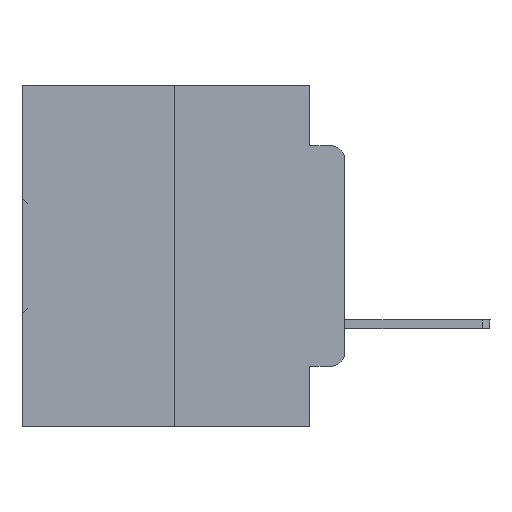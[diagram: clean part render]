
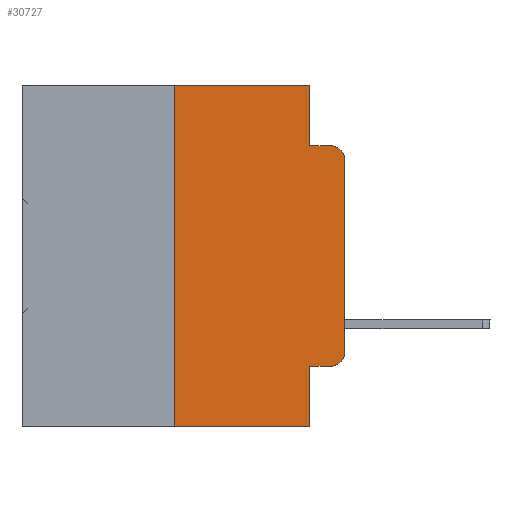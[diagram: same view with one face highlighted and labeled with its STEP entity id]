
A CAD part, left-side view. The second image highlights one B-rep face of the part: STEP entity #30727.
In plain terms, the highlighted planar face has unit normal (-1, 0, 0).
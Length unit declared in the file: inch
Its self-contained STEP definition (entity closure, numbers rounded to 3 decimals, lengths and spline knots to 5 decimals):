
#281 = LINE ( 'NONE', #11398, #8085 ) ;
#467 = ORIENTED_EDGE ( 'NONE', *, *, #11546, .F. ) ;
#2263 = VERTEX_POINT ( 'NONE', #15503 ) ;
#2699 = DIRECTION ( 'NONE',  ( 1., 0., 0. ) ) ;
#2722 = ORIENTED_EDGE ( 'NONE', *, *, #23367, .F. ) ;
#3305 = VECTOR ( 'NONE', #19633, 39.37008 ) ;
#3472 = DIRECTION ( 'NONE',  ( 0., -1., 0. ) ) ;
#3783 = CARTESIAN_POINT ( 'NONE',  ( 0., 0.25, 0. ) ) ;
#4512 = LINE ( 'NONE', #17762, #34932 ) ;
#5040 = ORIENTED_EDGE ( 'NONE', *, *, #28165, .T. ) ;
#6168 = CARTESIAN_POINT ( 'NONE',  ( 0., 0.25, 0. ) ) ;
#6306 = VERTEX_POINT ( 'NONE', #16588 ) ;
#7298 = EDGE_CURVE ( 'NONE', #8779, #32624, #9564, .T. ) ;
#7706 = AXIS2_PLACEMENT_3D ( 'NONE', #16877, #27318, #10704 ) ;
#7778 = DIRECTION ( 'NONE',  ( -1., 0., 0. ) ) ;
#7963 = EDGE_CURVE ( 'NONE', #8872, #6306, #30005, .T. ) ;
#8085 = VECTOR ( 'NONE', #22349, 39.37008 ) ;
#8494 = CARTESIAN_POINT ( 'NONE',  ( 0., 0.051, -0.4115 ) ) ;
#8779 = VERTEX_POINT ( 'NONE', #6168 ) ;
#8872 = VERTEX_POINT ( 'NONE', #8494 ) ;
#9047 = VECTOR ( 'NONE', #26353, 39.37008 ) ;
#9564 = LINE ( 'NONE', #23178, #12320 ) ;
#10517 = AXIS2_PLACEMENT_3D ( 'NONE', #12791, #2699, #31704 ) ;
#10704 = DIRECTION ( 'NONE',  ( 0., 0., -1. ) ) ;
#10722 = EDGE_CURVE ( 'NONE', #33563, #6306, #4512, .T. ) ;
#10736 = DIRECTION ( 'NONE',  ( 0., 0., -1. ) ) ;
#11398 = CARTESIAN_POINT ( 'NONE',  ( 0., 0., 0. ) ) ;
#11546 = EDGE_CURVE ( 'NONE', #18919, #2263, #17859, .T. ) ;
#12081 = DIRECTION ( 'NONE',  ( 0., 0., 1. ) ) ;
#12208 = DIRECTION ( 'NONE',  ( 0., -1., 0. ) ) ;
#12320 = VECTOR ( 'NONE', #12208, 39.37008 ) ;
#12494 = AXIS2_PLACEMENT_3D ( 'NONE', #26178, #7778, #26360 ) ;
#12791 = CARTESIAN_POINT ( 'NONE',  ( 0., 0.473, 0. ) ) ;
#12961 = EDGE_CURVE ( 'NONE', #33745, #2263, #23220, .T. ) ;
#13071 = ORIENTED_EDGE ( 'NONE', *, *, #12961, .T. ) ;
#13453 = EDGE_LOOP ( 'NONE', ( #5040, #13071, #467, #2722, #18790, #34384, #34401, #25281, #17009, #19165 ) ) ;
#13756 = VECTOR ( 'NONE', #12081, 39.37008 ) ;
#15111 = EDGE_CURVE ( 'NONE', #8872, #17032, #19899, .T. ) ;
#15503 = CARTESIAN_POINT ( 'NONE',  ( 0., 0.02, -0.0885 ) ) ;
#16416 = CARTESIAN_POINT ( 'NONE',  ( 0., 0., -0.3915 ) ) ;
#16588 = CARTESIAN_POINT ( 'NONE',  ( 0., 0.051, -0.5 ) ) ;
#16656 = EDGE_CURVE ( 'NONE', #17032, #18864, #22380, .T. ) ;
#16877 = CARTESIAN_POINT ( 'NONE',  ( 0., 0.02, -0.3915 ) ) ;
#17009 = ORIENTED_EDGE ( 'NONE', *, *, #15111, .T. ) ;
#17032 = VERTEX_POINT ( 'NONE', #30094 ) ;
#17762 = CARTESIAN_POINT ( 'NONE',  ( 0., 0.473, -0.5 ) ) ;
#17859 = LINE ( 'NONE', #18043, #9047 ) ;
#18043 = CARTESIAN_POINT ( 'NONE',  ( 0., 0.051, -0.0885 ) ) ;
#18284 = DIRECTION ( 'NONE',  ( 0., -1., 0. ) ) ;
#18790 = ORIENTED_EDGE ( 'NONE', *, *, #7298, .F. ) ;
#18864 = VERTEX_POINT ( 'NONE', #16416 ) ;
#18919 = VERTEX_POINT ( 'NONE', #31226 ) ;
#19165 = ORIENTED_EDGE ( 'NONE', *, *, #16656, .T. ) ;
#19633 = DIRECTION ( 'NONE',  ( 0., 0., -1. ) ) ;
#19899 = LINE ( 'NONE', #22567, #33051 ) ;
#21062 = CARTESIAN_POINT ( 'NONE',  ( 0., 0.25, -0.5 ) ) ;
#21919 = CARTESIAN_POINT ( 'NONE',  ( 0., 0.051, 0. ) ) ;
#22349 = DIRECTION ( 'NONE',  ( 0., 0., 1. ) ) ;
#22380 = CIRCLE ( 'NONE', #7706, 0.02 ) ;
#22567 = CARTESIAN_POINT ( 'NONE',  ( 0., 0.051, -0.4115 ) ) ;
#23178 = CARTESIAN_POINT ( 'NONE',  ( 0., 0.473, 0. ) ) ;
#23220 = CIRCLE ( 'NONE', #12494, 0.02 ) ;
#23367 = EDGE_CURVE ( 'NONE', #32624, #18919, #32363, .T. ) ;
#24358 = CARTESIAN_POINT ( 'NONE',  ( 0., 0.051, 0. ) ) ;
#24782 = CARTESIAN_POINT ( 'NONE',  ( 0., 0.051, 0. ) ) ;
#25281 = ORIENTED_EDGE ( 'NONE', *, *, #7963, .F. ) ;
#26178 = CARTESIAN_POINT ( 'NONE',  ( 0., 0.02, -0.1085 ) ) ;
#26353 = DIRECTION ( 'NONE',  ( 0., -1., 0. ) ) ;
#26360 = DIRECTION ( 'NONE',  ( 0., 0., -1. ) ) ;
#26413 = PLANE ( 'NONE',  #10517 ) ;
#27318 = DIRECTION ( 'NONE',  ( -1., 0., 0. ) ) ;
#28165 = EDGE_CURVE ( 'NONE', #18864, #33745, #281, .T. ) ;
#28332 = EDGE_CURVE ( 'NONE', #33563, #8779, #30641, .T. ) ;
#29588 = VECTOR ( 'NONE', #10736, 39.37008 ) ;
#30005 = LINE ( 'NONE', #24358, #29588 ) ;
#30094 = CARTESIAN_POINT ( 'NONE',  ( 0., 0.02, -0.4115 ) ) ;
#30641 = LINE ( 'NONE', #3783, #13756 ) ;
#30727 = ADVANCED_FACE ( 'NONE', ( #34863 ), #26413, .F. ) ;
#31226 = CARTESIAN_POINT ( 'NONE',  ( 0., 0.051, -0.0885 ) ) ;
#31704 = DIRECTION ( 'NONE',  ( 0., 0., -1. ) ) ;
#32363 = LINE ( 'NONE', #24782, #3305 ) ;
#32624 = VERTEX_POINT ( 'NONE', #21919 ) ;
#33051 = VECTOR ( 'NONE', #3472, 39.37008 ) ;
#33175 = CARTESIAN_POINT ( 'NONE',  ( 0., 0., -0.1085 ) ) ;
#33563 = VERTEX_POINT ( 'NONE', #21062 ) ;
#33745 = VERTEX_POINT ( 'NONE', #33175 ) ;
#34384 = ORIENTED_EDGE ( 'NONE', *, *, #28332, .F. ) ;
#34401 = ORIENTED_EDGE ( 'NONE', *, *, #10722, .T. ) ;
#34863 = FACE_OUTER_BOUND ( 'NONE', #13453, .T. ) ;
#34932 = VECTOR ( 'NONE', #18284, 39.37008 ) ;
